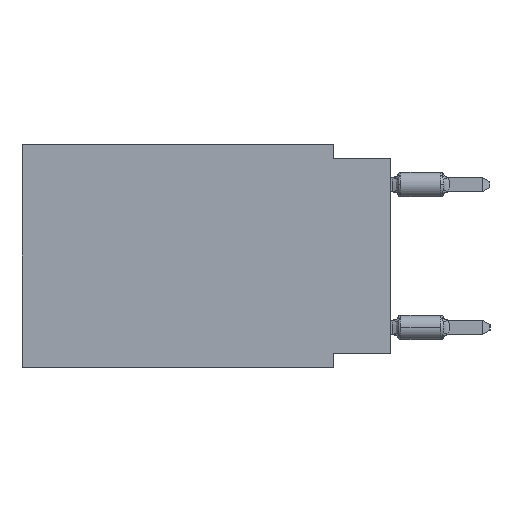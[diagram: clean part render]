
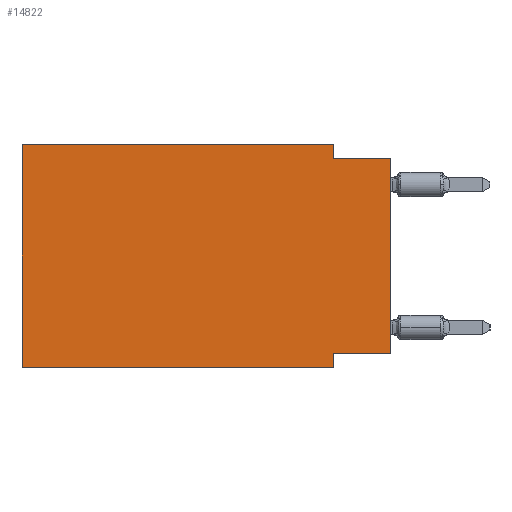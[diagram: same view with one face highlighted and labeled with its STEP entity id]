
A CAD part, left-side view. The second image highlights one B-rep face of the part: STEP entity #14822.
In plain terms, the highlighted planar face has unit normal (-1, 0, 0).
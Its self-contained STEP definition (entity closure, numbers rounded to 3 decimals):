
#337 = CARTESIAN_POINT ( 'NONE',  ( 0., 2.54, -9.271 ) ) ;
#637 = ORIENTED_EDGE ( 'NONE', *, *, #13166, .F. ) ;
#2159 = CARTESIAN_POINT ( 'NONE',  ( 0., 16.383, 0. ) ) ;
#2538 = DIRECTION ( 'NONE',  ( 0., -1., 0. ) ) ;
#2763 = CARTESIAN_POINT ( 'NONE',  ( 0., 16.383, -9.906 ) ) ;
#2929 = ORIENTED_EDGE ( 'NONE', *, *, #12758, .T. ) ;
#3069 = LINE ( 'NONE', #24617, #18812 ) ;
#3244 = VERTEX_POINT ( 'NONE', #6215 ) ;
#3629 = EDGE_CURVE ( 'NONE', #22649, #3244, #25383, .T. ) ;
#3730 = VERTEX_POINT ( 'NONE', #24086 ) ;
#3827 = LINE ( 'NONE', #9958, #3996 ) ;
#3996 = VECTOR ( 'NONE', #6044, 1000. ) ;
#4021 = EDGE_CURVE ( 'NONE', #7833, #13317, #5628, .T. ) ;
#4442 = VECTOR ( 'NONE', #13740, 1000. ) ;
#4814 = VECTOR ( 'NONE', #20268, 1000. ) ;
#5466 = EDGE_CURVE ( 'NONE', #24825, #22618, #16599, .T. ) ;
#5483 = VECTOR ( 'NONE', #2538, 1000. ) ;
#5628 = LINE ( 'NONE', #21701, #7682 ) ;
#6044 = DIRECTION ( 'NONE',  ( 0., -1., 0. ) ) ;
#6215 = CARTESIAN_POINT ( 'NONE',  ( 0., 2.54, -0.635 ) ) ;
#6652 = ORIENTED_EDGE ( 'NONE', *, *, #9332, .T. ) ;
#7100 = AXIS2_PLACEMENT_3D ( 'NONE', #19460, #21678, #17506 ) ;
#7682 = VECTOR ( 'NONE', #23527, 1000. ) ;
#7722 = CARTESIAN_POINT ( 'NONE',  ( 0., 0., 0. ) ) ;
#7833 = VERTEX_POINT ( 'NONE', #337 ) ;
#8869 = EDGE_CURVE ( 'NONE', #22618, #22649, #3827, .T. ) ;
#9332 = EDGE_CURVE ( 'NONE', #19810, #3730, #17527, .T. ) ;
#9409 = PLANE ( 'NONE',  #7100 ) ;
#9533 = ORIENTED_EDGE ( 'NONE', *, *, #3629, .F. ) ;
#9958 = CARTESIAN_POINT ( 'NONE',  ( 0., 16.383, 0. ) ) ;
#11755 = ORIENTED_EDGE ( 'NONE', *, *, #5466, .F. ) ;
#12758 = EDGE_CURVE ( 'NONE', #24825, #13317, #3069, .T. ) ;
#13166 = EDGE_CURVE ( 'NONE', #3244, #3730, #14780, .T. ) ;
#13317 = VERTEX_POINT ( 'NONE', #17139 ) ;
#13740 = DIRECTION ( 'NONE',  ( 0., 0., 1. ) ) ;
#14200 = ORIENTED_EDGE ( 'NONE', *, *, #17293, .F. ) ;
#14411 = CARTESIAN_POINT ( 'NONE',  ( 0., 0., -0.635 ) ) ;
#14780 = LINE ( 'NONE', #14411, #5483 ) ;
#14822 = ADVANCED_FACE ( 'NONE', ( #23642 ), #9409, .F. ) ;
#16428 = VECTOR ( 'NONE', #23432, 1000. ) ;
#16599 = LINE ( 'NONE', #24566, #4814 ) ;
#17139 = CARTESIAN_POINT ( 'NONE',  ( 0., 2.54, -9.906 ) ) ;
#17293 = EDGE_CURVE ( 'NONE', #19810, #7833, #19885, .T. ) ;
#17451 = EDGE_LOOP ( 'NONE', ( #6652, #637, #9533, #23917, #11755, #2929, #24048, #14200 ) ) ;
#17506 = DIRECTION ( 'NONE',  ( 0., 0., -1. ) ) ;
#17527 = LINE ( 'NONE', #7722, #4442 ) ;
#18812 = VECTOR ( 'NONE', #20824, 1000. ) ;
#19460 = CARTESIAN_POINT ( 'NONE',  ( 0., 16.383, 0. ) ) ;
#19810 = VERTEX_POINT ( 'NONE', #20668 ) ;
#19885 = LINE ( 'NONE', #22244, #25358 ) ;
#20268 = DIRECTION ( 'NONE',  ( 0., 0., 1. ) ) ;
#20668 = CARTESIAN_POINT ( 'NONE',  ( 0., 0., -9.271 ) ) ;
#20824 = DIRECTION ( 'NONE',  ( 0., -1., 0. ) ) ;
#20955 = CARTESIAN_POINT ( 'NONE',  ( 0., 2.54, 0. ) ) ;
#21678 = DIRECTION ( 'NONE',  ( 1., 0., 0. ) ) ;
#21701 = CARTESIAN_POINT ( 'NONE',  ( 0., 2.54, -9.906 ) ) ;
#22119 = DIRECTION ( 'NONE',  ( 0., 1., 0. ) ) ;
#22244 = CARTESIAN_POINT ( 'NONE',  ( 0., 0., -9.271 ) ) ;
#22384 = CARTESIAN_POINT ( 'NONE',  ( 0., 2.54, 0. ) ) ;
#22618 = VERTEX_POINT ( 'NONE', #2159 ) ;
#22649 = VERTEX_POINT ( 'NONE', #22384 ) ;
#23432 = DIRECTION ( 'NONE',  ( 0., 0., -1. ) ) ;
#23527 = DIRECTION ( 'NONE',  ( 0., 0., -1. ) ) ;
#23642 = FACE_OUTER_BOUND ( 'NONE', #17451, .T. ) ;
#23917 = ORIENTED_EDGE ( 'NONE', *, *, #8869, .F. ) ;
#24048 = ORIENTED_EDGE ( 'NONE', *, *, #4021, .F. ) ;
#24086 = CARTESIAN_POINT ( 'NONE',  ( 0., 0., -0.635 ) ) ;
#24566 = CARTESIAN_POINT ( 'NONE',  ( 0., 16.383, 0. ) ) ;
#24617 = CARTESIAN_POINT ( 'NONE',  ( 0., 16.383, -9.906 ) ) ;
#24825 = VERTEX_POINT ( 'NONE', #2763 ) ;
#25358 = VECTOR ( 'NONE', #22119, 1000. ) ;
#25383 = LINE ( 'NONE', #20955, #16428 ) ;
